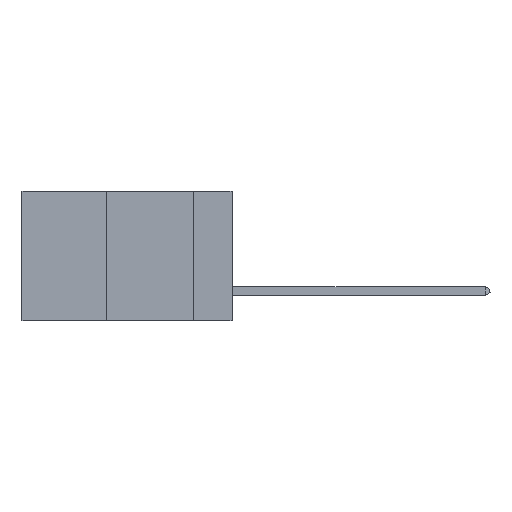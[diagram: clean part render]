
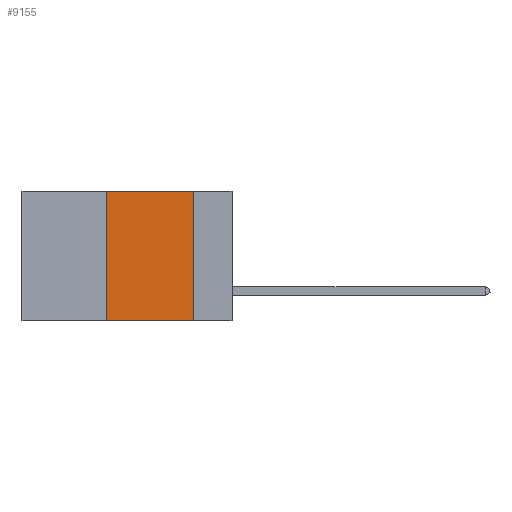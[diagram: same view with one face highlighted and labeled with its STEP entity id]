
A CAD part, left-side view. The second image highlights one B-rep face of the part: STEP entity #9155.
In plain terms, the highlighted planar face has unit normal (-1, 0, 0).
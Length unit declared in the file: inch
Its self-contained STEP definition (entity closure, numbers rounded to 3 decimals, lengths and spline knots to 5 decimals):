
#126 = EDGE_LOOP ( 'NONE', ( #8665, #3755, #11951, #4488 ) ) ;
#745 = DIRECTION ( 'NONE',  ( 1., 0., 0. ) ) ;
#1212 = CARTESIAN_POINT ( 'NONE',  ( 0., 0.11, 0. ) ) ;
#1425 = DIRECTION ( 'NONE',  ( 0., 0., 1. ) ) ;
#2104 = DIRECTION ( 'NONE',  ( 0., 0., -1. ) ) ;
#3209 = CARTESIAN_POINT ( 'NONE',  ( 0., 0.36, 0. ) ) ;
#3755 = ORIENTED_EDGE ( 'NONE', *, *, #11207, .F. ) ;
#4378 = CARTESIAN_POINT ( 'NONE',  ( 0., 0.11, -0.37 ) ) ;
#4488 = ORIENTED_EDGE ( 'NONE', *, *, #10879, .T. ) ;
#5649 = FACE_OUTER_BOUND ( 'NONE', #126, .T. ) ;
#5749 = VECTOR ( 'NONE', #8613, 39.37008 ) ;
#5858 = VERTEX_POINT ( 'NONE', #10193 ) ;
#6045 = LINE ( 'NONE', #6871, #5749 ) ;
#6182 = LINE ( 'NONE', #1212, #12277 ) ;
#6478 = CARTESIAN_POINT ( 'NONE',  ( 0., 0.6, 0. ) ) ;
#6871 = CARTESIAN_POINT ( 'NONE',  ( 0., 0.6, 0. ) ) ;
#6967 = VERTEX_POINT ( 'NONE', #8282 ) ;
#8282 = CARTESIAN_POINT ( 'NONE',  ( 0., 0.11, 0. ) ) ;
#8449 = LINE ( 'NONE', #3209, #10360 ) ;
#8575 = CARTESIAN_POINT ( 'NONE',  ( 0., 0.36, 0. ) ) ;
#8613 = DIRECTION ( 'NONE',  ( 0., -1., 0. ) ) ;
#8665 = ORIENTED_EDGE ( 'NONE', *, *, #11862, .F. ) ;
#9155 = ADVANCED_FACE ( 'NONE', ( #5649 ), #12204, .F. ) ;
#9183 = DIRECTION ( 'NONE',  ( 0., 0., -1. ) ) ;
#10193 = CARTESIAN_POINT ( 'NONE',  ( 0., 0.36, -0.37 ) ) ;
#10292 = EDGE_CURVE ( 'NONE', #5858, #11150, #8449, .T. ) ;
#10337 = LINE ( 'NONE', #10931, #11101 ) ;
#10360 = VECTOR ( 'NONE', #1425, 39.37008 ) ;
#10853 = VERTEX_POINT ( 'NONE', #4378 ) ;
#10879 = EDGE_CURVE ( 'NONE', #5858, #10853, #10337, .T. ) ;
#10931 = CARTESIAN_POINT ( 'NONE',  ( 0., 0.6, -0.37 ) ) ;
#11101 = VECTOR ( 'NONE', #11952, 39.37008 ) ;
#11150 = VERTEX_POINT ( 'NONE', #8575 ) ;
#11207 = EDGE_CURVE ( 'NONE', #11150, #6967, #6045, .T. ) ;
#11431 = AXIS2_PLACEMENT_3D ( 'NONE', #6478, #745, #9183 ) ;
#11862 = EDGE_CURVE ( 'NONE', #6967, #10853, #6182, .T. ) ;
#11951 = ORIENTED_EDGE ( 'NONE', *, *, #10292, .F. ) ;
#11952 = DIRECTION ( 'NONE',  ( 0., -1., 0. ) ) ;
#12204 = PLANE ( 'NONE',  #11431 ) ;
#12277 = VECTOR ( 'NONE', #2104, 39.37008 ) ;
